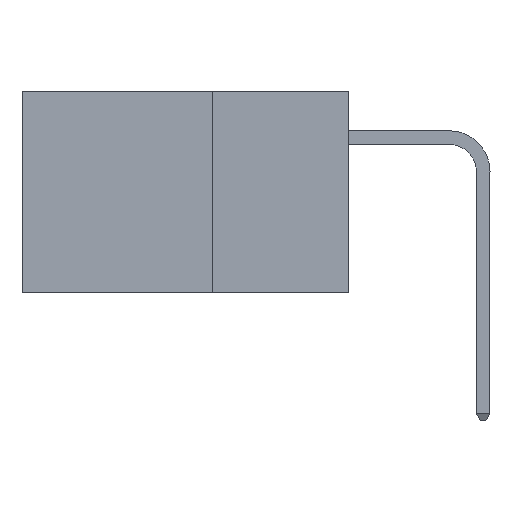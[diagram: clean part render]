
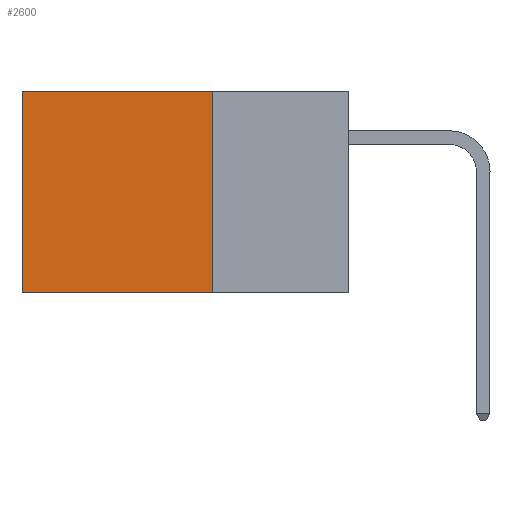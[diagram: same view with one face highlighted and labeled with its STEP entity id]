
A CAD part, left-side view. The second image highlights one B-rep face of the part: STEP entity #2600.
In plain terms, the highlighted planar face has unit normal (-1, 0, 0).
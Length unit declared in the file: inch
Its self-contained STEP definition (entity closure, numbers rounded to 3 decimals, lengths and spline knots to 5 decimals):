
#82 = ORIENTED_EDGE ( 'NONE', *, *, #20194, .T. ) ;
#525 = CARTESIAN_POINT ( 'NONE',  ( 0.2875, 0.6, 0. ) ) ;
#529 = VECTOR ( 'NONE', #16500, 39.37008 ) ;
#2600 = ADVANCED_FACE ( 'NONE', ( #22987 ), #13439, .F. ) ;
#7599 = CARTESIAN_POINT ( 'NONE',  ( 0.2875, 0.6, -0.37 ) ) ;
#7940 = VECTOR ( 'NONE', #31270, 39.37008 ) ;
#8449 = ORIENTED_EDGE ( 'NONE', *, *, #22391, .T. ) ;
#9127 = AXIS2_PLACEMENT_3D ( 'NONE', #32406, #24009, #34796 ) ;
#9172 = EDGE_LOOP ( 'NONE', ( #82, #18723, #35316, #8449 ) ) ;
#10171 = VECTOR ( 'NONE', #24587, 39.37008 ) ;
#11093 = CARTESIAN_POINT ( 'NONE',  ( 0.2875, 0.25, -0.37 ) ) ;
#13109 = LINE ( 'NONE', #28527, #7940 ) ;
#13439 = PLANE ( 'NONE',  #9127 ) ;
#14055 = EDGE_CURVE ( 'NONE', #14069, #25949, #14284, .T. ) ;
#14069 = VERTEX_POINT ( 'NONE', #34909 ) ;
#14284 = LINE ( 'NONE', #32157, #529 ) ;
#16500 = DIRECTION ( 'NONE',  ( 0., 0., -1. ) ) ;
#17440 = LINE ( 'NONE', #30116, #10171 ) ;
#18723 = ORIENTED_EDGE ( 'NONE', *, *, #24448, .F. ) ;
#20194 = EDGE_CURVE ( 'NONE', #23667, #23924, #31988, .T. ) ;
#22391 = EDGE_CURVE ( 'NONE', #14069, #23667, #17440, .T. ) ;
#22987 = FACE_OUTER_BOUND ( 'NONE', #9172, .T. ) ;
#23667 = VERTEX_POINT ( 'NONE', #525 ) ;
#23924 = VERTEX_POINT ( 'NONE', #7599 ) ;
#24009 = DIRECTION ( 'NONE',  ( 1., 0., 0. ) ) ;
#24448 = EDGE_CURVE ( 'NONE', #25949, #23924, #13109, .T. ) ;
#24587 = DIRECTION ( 'NONE',  ( 0., 1., 0. ) ) ;
#25949 = VERTEX_POINT ( 'NONE', #11093 ) ;
#26063 = VECTOR ( 'NONE', #34234, 39.37008 ) ;
#28527 = CARTESIAN_POINT ( 'NONE',  ( 0.2875, 0.25, -0.37 ) ) ;
#30116 = CARTESIAN_POINT ( 'NONE',  ( 0.2875, 0.25, 0. ) ) ;
#31270 = DIRECTION ( 'NONE',  ( 0., 1., 0. ) ) ;
#31831 = CARTESIAN_POINT ( 'NONE',  ( 0.2875, 0.6, 0. ) ) ;
#31988 = LINE ( 'NONE', #31831, #26063 ) ;
#32157 = CARTESIAN_POINT ( 'NONE',  ( 0.2875, 0.25, 0. ) ) ;
#32406 = CARTESIAN_POINT ( 'NONE',  ( 0.2875, 0.25, 0. ) ) ;
#34234 = DIRECTION ( 'NONE',  ( 0., 0., -1. ) ) ;
#34796 = DIRECTION ( 'NONE',  ( 0., 0., -1. ) ) ;
#34909 = CARTESIAN_POINT ( 'NONE',  ( 0.2875, 0.25, 0. ) ) ;
#35316 = ORIENTED_EDGE ( 'NONE', *, *, #14055, .F. ) ;
